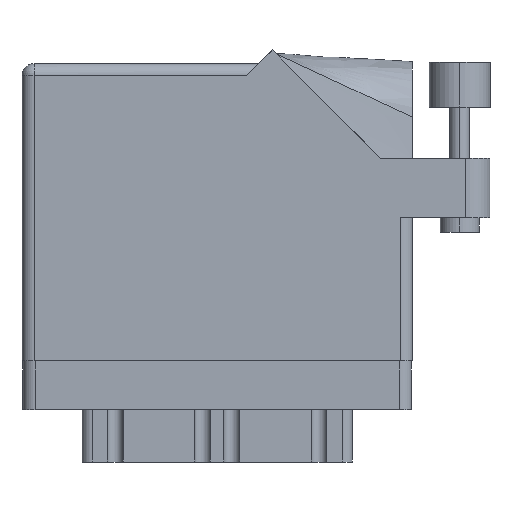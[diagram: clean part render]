
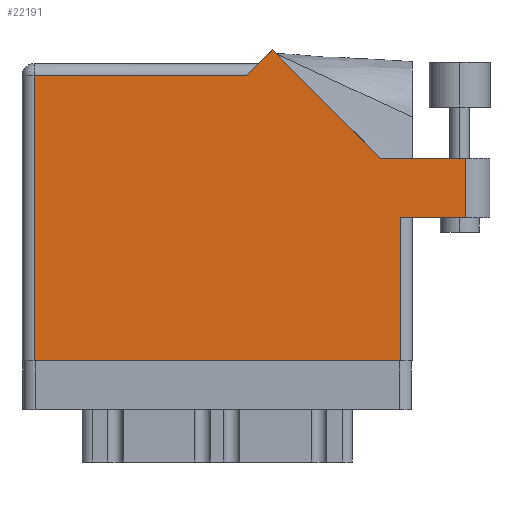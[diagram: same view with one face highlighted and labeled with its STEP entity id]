
A CAD part, front view. The second image highlights one B-rep face of the part: STEP entity #22191.
In plain terms, the highlighted face is planar.
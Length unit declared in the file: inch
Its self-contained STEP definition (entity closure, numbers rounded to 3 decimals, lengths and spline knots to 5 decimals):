
#348 = VERTEX_POINT ( 'NONE', #21282 ) ;
#1237 = LINE ( 'NONE', #9460, #11863 ) ;
#1362 = DIRECTION ( 'NONE',  ( -1., 0., 0. ) ) ;
#1411 = CARTESIAN_POINT ( 'NONE',  ( 1.948, 0., 0. ) ) ;
#1782 = VERTEX_POINT ( 'NONE', #24895 ) ;
#2033 = VERTEX_POINT ( 'NONE', #21192 ) ;
#2120 = DIRECTION ( 'NONE',  ( 1., 0., 0. ) ) ;
#2709 = ORIENTED_EDGE ( 'NONE', *, *, #18158, .T. ) ;
#3269 = DIRECTION ( 'NONE',  ( 0., 1., 0. ) ) ;
#3553 = EDGE_LOOP ( 'NONE', ( #34558, #17510, #9891, #15336, #6950, #19019, #5963, #2709, #33512 ) ) ;
#5120 = AXIS2_PLACEMENT_3D ( 'NONE', #9420, #30996, #1362 ) ;
#5617 = CARTESIAN_POINT ( 'NONE',  ( 1.948, 0.737, 0. ) ) ;
#5963 = ORIENTED_EDGE ( 'NONE', *, *, #17316, .T. ) ;
#6194 = VERTEX_POINT ( 'NONE', #23639 ) ;
#6950 = ORIENTED_EDGE ( 'NONE', *, *, #15699, .T. ) ;
#7996 = VERTEX_POINT ( 'NONE', #21820 ) ;
#8863 = CARTESIAN_POINT ( 'NONE',  ( 2.41, 1.044, 0. ) ) ;
#9420 = CARTESIAN_POINT ( 'NONE',  ( 0., 1.53, 0. ) ) ;
#9460 = CARTESIAN_POINT ( 'NONE',  ( 2.285, 1.044, 0. ) ) ;
#9891 = ORIENTED_EDGE ( 'NONE', *, *, #17794, .T. ) ;
#10676 = VECTOR ( 'NONE', #24339, 39.37008 ) ;
#11863 = VECTOR ( 'NONE', #20151, 39.37008 ) ;
#13821 = VECTOR ( 'NONE', #2120, 39.37008 ) ;
#13884 = CARTESIAN_POINT ( 'NONE',  ( 0., 0., 0. ) ) ;
#13939 = LINE ( 'NONE', #22185, #18534 ) ;
#14318 = LINE ( 'NONE', #24499, #10676 ) ;
#14637 = LINE ( 'NONE', #28493, #20507 ) ;
#14668 = FACE_OUTER_BOUND ( 'NONE', #3553, .T. ) ;
#15183 = CARTESIAN_POINT ( 'NONE',  ( 1.28771, 1.60071, 0. ) ) ;
#15336 = ORIENTED_EDGE ( 'NONE', *, *, #16978, .T. ) ;
#15699 = EDGE_CURVE ( 'NONE', #30240, #1782, #28238, .T. ) ;
#15789 = LINE ( 'NONE', #25951, #13821 ) ;
#16407 = EDGE_CURVE ( 'NONE', #26610, #20247, #13939, .T. ) ;
#16978 = EDGE_CURVE ( 'NONE', #24232, #30240, #20039, .T. ) ;
#17268 = DIRECTION ( 'NONE',  ( -1., 0., 0. ) ) ;
#17316 = EDGE_CURVE ( 'NONE', #6194, #348, #14318, .T. ) ;
#17510 = ORIENTED_EDGE ( 'NONE', *, *, #25385, .T. ) ;
#17794 = EDGE_CURVE ( 'NONE', #7996, #24232, #22005, .T. ) ;
#18158 = EDGE_CURVE ( 'NONE', #348, #26610, #24254, .T. ) ;
#18534 = VECTOR ( 'NONE', #3269, 39.37008 ) ;
#19019 = ORIENTED_EDGE ( 'NONE', *, *, #19231, .T. ) ;
#19231 = EDGE_CURVE ( 'NONE', #1782, #6194, #14637, .T. ) ;
#19306 = VECTOR ( 'NONE', #19550, 39.37008 ) ;
#19550 = DIRECTION ( 'NONE',  ( -1., 0., 0. ) ) ;
#20039 = LINE ( 'NONE', #30923, #30323 ) ;
#20098 = EDGE_CURVE ( 'NONE', #20247, #2033, #15789, .T. ) ;
#20151 = DIRECTION ( 'NONE',  ( 0., 1., 0. ) ) ;
#20167 = CARTESIAN_POINT ( 'NONE',  ( 1.217, 1.53, 0. ) ) ;
#20247 = VERTEX_POINT ( 'NONE', #5617 ) ;
#20507 = VECTOR ( 'NONE', #17268, 39.37008 ) ;
#21192 = CARTESIAN_POINT ( 'NONE',  ( 2.285, 0.737, 0. ) ) ;
#21282 = CARTESIAN_POINT ( 'NONE',  ( 0.062, 0., 0. ) ) ;
#21820 = CARTESIAN_POINT ( 'NONE',  ( 2.285, 1.044, 0. ) ) ;
#22005 = LINE ( 'NONE', #8863, #19306 ) ;
#22185 = CARTESIAN_POINT ( 'NONE',  ( 1.948, 0.737, 0. ) ) ;
#22191 = ADVANCED_FACE ( 'NONE', ( #14668 ), #33620, .F. ) ;
#23639 = CARTESIAN_POINT ( 'NONE',  ( 0.062, 1.468, 0. ) ) ;
#24232 = VERTEX_POINT ( 'NONE', #29544 ) ;
#24254 = LINE ( 'NONE', #13884, #29985 ) ;
#24339 = DIRECTION ( 'NONE',  ( 0., -1., 0. ) ) ;
#24499 = CARTESIAN_POINT ( 'NONE',  ( 0.062, 0., 0. ) ) ;
#24590 = DIRECTION ( 'NONE',  ( 1., 0., 0. ) ) ;
#24895 = CARTESIAN_POINT ( 'NONE',  ( 1.155, 1.468, 0. ) ) ;
#25385 = EDGE_CURVE ( 'NONE', #2033, #7996, #1237, .T. ) ;
#25951 = CARTESIAN_POINT ( 'NONE',  ( 2.01, 0.737, 0. ) ) ;
#26292 = DIRECTION ( 'NONE',  ( -0.707, -0.707, 0. ) ) ;
#26610 = VERTEX_POINT ( 'NONE', #1411 ) ;
#28238 = LINE ( 'NONE', #20167, #29236 ) ;
#28493 = CARTESIAN_POINT ( 'NONE',  ( 0., 1.468, 0. ) ) ;
#29236 = VECTOR ( 'NONE', #26292, 39.37008 ) ;
#29544 = CARTESIAN_POINT ( 'NONE',  ( 1.84442, 1.044, 0. ) ) ;
#29985 = VECTOR ( 'NONE', #24590, 39.37008 ) ;
#30240 = VERTEX_POINT ( 'NONE', #15183 ) ;
#30323 = VECTOR ( 'NONE', #33373, 39.37008 ) ;
#30923 = CARTESIAN_POINT ( 'NONE',  ( 1.84442, 1.044, 0. ) ) ;
#30996 = DIRECTION ( 'NONE',  ( 0., 0., -1. ) ) ;
#33373 = DIRECTION ( 'NONE',  ( -0.707, 0.707, 0. ) ) ;
#33512 = ORIENTED_EDGE ( 'NONE', *, *, #16407, .T. ) ;
#33620 = PLANE ( 'NONE',  #5120 ) ;
#34558 = ORIENTED_EDGE ( 'NONE', *, *, #20098, .T. ) ;
